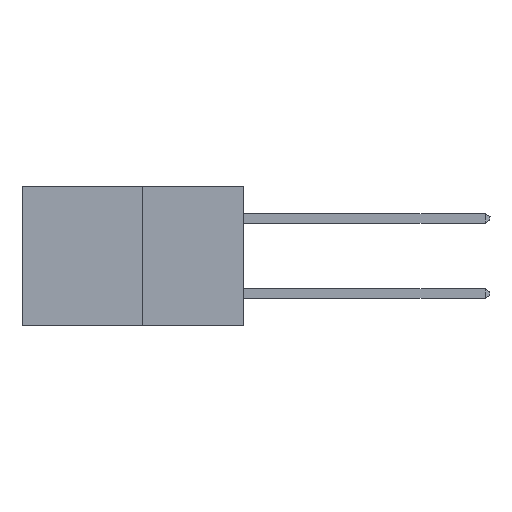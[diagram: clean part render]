
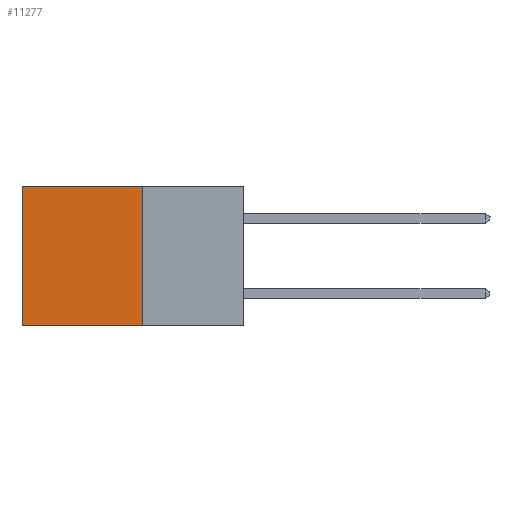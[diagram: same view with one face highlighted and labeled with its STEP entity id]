
A CAD part, left-side view. The second image highlights one B-rep face of the part: STEP entity #11277.
In plain terms, the highlighted planar face has unit normal (-1, 0, 0).
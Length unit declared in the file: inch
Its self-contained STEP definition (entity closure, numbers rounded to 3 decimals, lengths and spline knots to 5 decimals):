
#997 = DIRECTION ( 'NONE',  ( 1., 0., 0. ) ) ;
#1245 = ORIENTED_EDGE ( 'NONE', *, *, #16135, .F. ) ;
#2662 = CARTESIAN_POINT ( 'NONE',  ( 0.277, 0.27, -0.37 ) ) ;
#2881 = CARTESIAN_POINT ( 'NONE',  ( 0.277, 0.27, -0.37 ) ) ;
#3251 = CARTESIAN_POINT ( 'NONE',  ( 0.277, 0.27, 0. ) ) ;
#3258 = EDGE_CURVE ( 'NONE', #15945, #10292, #7180, .T. ) ;
#4025 = CARTESIAN_POINT ( 'NONE',  ( 0.277, 0.59, -0.37 ) ) ;
#4215 = ORIENTED_EDGE ( 'NONE', *, *, #14432, .F. ) ;
#4320 = ORIENTED_EDGE ( 'NONE', *, *, #5948, .T. ) ;
#4618 = DIRECTION ( 'NONE',  ( 0., 0., -1. ) ) ;
#4635 = DIRECTION ( 'NONE',  ( 0., 1., 0. ) ) ;
#4878 = DIRECTION ( 'NONE',  ( 0., 1., 0. ) ) ;
#5707 = VECTOR ( 'NONE', #19829, 39.37008 ) ;
#5948 = EDGE_CURVE ( 'NONE', #10292, #15828, #24588, .T. ) ;
#7180 = LINE ( 'NONE', #3251, #17842 ) ;
#7703 = VECTOR ( 'NONE', #4618, 39.37008 ) ;
#8977 = LINE ( 'NONE', #19565, #19614 ) ;
#10292 = VERTEX_POINT ( 'NONE', #17152 ) ;
#10355 = FACE_OUTER_BOUND ( 'NONE', #21612, .T. ) ;
#11277 = ADVANCED_FACE ( 'NONE', ( #10355 ), #24367, .F. ) ;
#11371 = LINE ( 'NONE', #2662, #5707 ) ;
#11696 = CARTESIAN_POINT ( 'NONE',  ( 0.277, 0.27, -0.37 ) ) ;
#12609 = CARTESIAN_POINT ( 'NONE',  ( 0.277, 0.27, 0. ) ) ;
#14432 = EDGE_CURVE ( 'NONE', #15945, #17672, #11371, .T. ) ;
#15828 = VERTEX_POINT ( 'NONE', #22898 ) ;
#15945 = VERTEX_POINT ( 'NONE', #12609 ) ;
#15990 = DIRECTION ( 'NONE',  ( 0., 0., -1. ) ) ;
#16135 = EDGE_CURVE ( 'NONE', #17672, #15828, #8977, .T. ) ;
#16492 = ORIENTED_EDGE ( 'NONE', *, *, #3258, .T. ) ;
#16670 = AXIS2_PLACEMENT_3D ( 'NONE', #11696, #997, #15990 ) ;
#17152 = CARTESIAN_POINT ( 'NONE',  ( 0.277, 0.59, 0. ) ) ;
#17672 = VERTEX_POINT ( 'NONE', #2881 ) ;
#17842 = VECTOR ( 'NONE', #4878, 39.37008 ) ;
#19565 = CARTESIAN_POINT ( 'NONE',  ( 0.277, 0.27, -0.37 ) ) ;
#19614 = VECTOR ( 'NONE', #4635, 39.37008 ) ;
#19829 = DIRECTION ( 'NONE',  ( 0., 0., -1. ) ) ;
#21612 = EDGE_LOOP ( 'NONE', ( #4320, #1245, #4215, #16492 ) ) ;
#22898 = CARTESIAN_POINT ( 'NONE',  ( 0.277, 0.59, -0.37 ) ) ;
#24367 = PLANE ( 'NONE',  #16670 ) ;
#24588 = LINE ( 'NONE', #4025, #7703 ) ;
